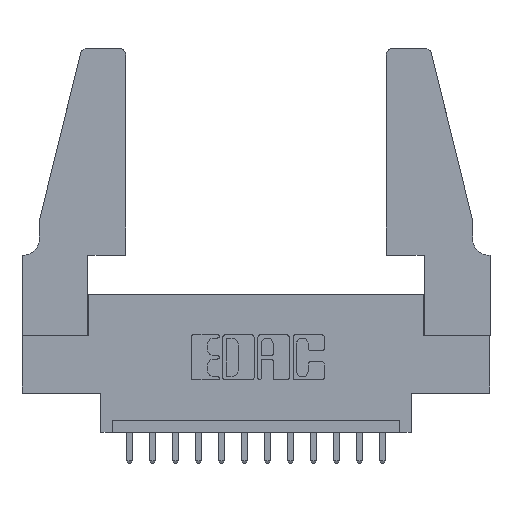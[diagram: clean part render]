
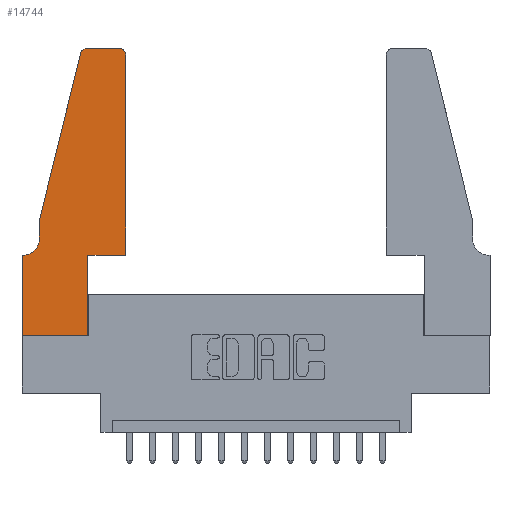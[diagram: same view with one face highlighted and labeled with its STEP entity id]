
A CAD part, top view. The second image highlights one B-rep face of the part: STEP entity #14744.
In plain terms, the highlighted planar face has unit normal (0, 0, 1).
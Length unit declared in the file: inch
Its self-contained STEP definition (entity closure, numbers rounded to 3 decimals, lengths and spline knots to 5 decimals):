
#138 = DIRECTION ( 'NONE',  ( 0., 0., 1. ) ) ;
#202 = ORIENTED_EDGE ( 'NONE', *, *, #7635, .T. ) ;
#237 = LINE ( 'NONE', #12779, #1346 ) ;
#288 = AXIS2_PLACEMENT_3D ( 'NONE', #14298, #138, #10239 ) ;
#647 = VECTOR ( 'NONE', #1321, 39.37008 ) ;
#767 = EDGE_CURVE ( 'NONE', #5536, #14315, #11030, .T. ) ;
#823 = DIRECTION ( 'NONE',  ( 0., 0., -1. ) ) ;
#906 = VECTOR ( 'NONE', #11679, 39.37008 ) ;
#923 = CARTESIAN_POINT ( 'NONE',  ( 0.0055, 0.42, 0.37 ) ) ;
#1123 = PLANE ( 'NONE',  #288 ) ;
#1277 = DIRECTION ( 'NONE',  ( -1., 0., 0. ) ) ;
#1321 = DIRECTION ( 'NONE',  ( 0., 1., 0. ) ) ;
#1346 = VECTOR ( 'NONE', #3264, 39.37008 ) ;
#1425 = CARTESIAN_POINT ( 'NONE',  ( 0.4505, 0.35, 0.37 ) ) ;
#1494 = DIRECTION ( 'NONE',  ( 0., 0., 1. ) ) ;
#1525 = DIRECTION ( 'NONE',  ( 1., 0., 0. ) ) ;
#1696 = CARTESIAN_POINT ( 'NONE',  ( 0.0055, 0.35, 0.37 ) ) ;
#1707 = CARTESIAN_POINT ( 'NONE',  ( 0.0755, 0.5, 0.37 ) ) ;
#1732 = AXIS2_PLACEMENT_3D ( 'NONE', #12116, #1494, #11066 ) ;
#1877 = VERTEX_POINT ( 'NONE', #15377 ) ;
#1930 = DIRECTION ( 'NONE',  ( -1., 0., 0. ) ) ;
#2265 = EDGE_CURVE ( 'NONE', #14378, #5536, #12870, .T. ) ;
#2634 = AXIS2_PLACEMENT_3D ( 'NONE', #923, #823, #1930 ) ;
#2693 = EDGE_CURVE ( 'NONE', #3538, #1877, #11007, .T. ) ;
#2780 = CARTESIAN_POINT ( 'NONE',  ( 0., 0., 0.37 ) ) ;
#2861 = VECTOR ( 'NONE', #1277, 39.37008 ) ;
#2972 = CARTESIAN_POINT ( 'NONE',  ( 0., 0., 0.37 ) ) ;
#3026 = CARTESIAN_POINT ( 'NONE',  ( 0.25487, 1.22718, 0.37 ) ) ;
#3035 = ORIENTED_EDGE ( 'NONE', *, *, #10656, .T. ) ;
#3264 = DIRECTION ( 'NONE',  ( 0., -1., 0. ) ) ;
#3538 = VERTEX_POINT ( 'NONE', #13537 ) ;
#4671 = CARTESIAN_POINT ( 'NONE',  ( 0.2865, 0.35, 0.37 ) ) ;
#4835 = CARTESIAN_POINT ( 'NONE',  ( 0.2865, 0., 0.37 ) ) ;
#4898 = ORIENTED_EDGE ( 'NONE', *, *, #13593, .T. ) ;
#5026 = VERTEX_POINT ( 'NONE', #4835 ) ;
#5220 = CARTESIAN_POINT ( 'NONE',  ( 0.4505, 0.35, 0.37 ) ) ;
#5362 = ORIENTED_EDGE ( 'NONE', *, *, #5808, .T. ) ;
#5449 = DIRECTION ( 'NONE',  ( -0.239, -0.971, 0. ) ) ;
#5536 = VERTEX_POINT ( 'NONE', #5220 ) ;
#5580 = VERTEX_POINT ( 'NONE', #10053 ) ;
#5808 = EDGE_CURVE ( 'NONE', #6667, #7899, #237, .T. ) ;
#5862 = DIRECTION ( 'NONE',  ( 0., 1., 0. ) ) ;
#6001 = LINE ( 'NONE', #6035, #2861 ) ;
#6035 = CARTESIAN_POINT ( 'NONE',  ( 0.2605, 1.25, 0.37 ) ) ;
#6037 = EDGE_CURVE ( 'NONE', #7899, #5026, #14707, .T. ) ;
#6152 = ORIENTED_EDGE ( 'NONE', *, *, #15047, .T. ) ;
#6179 = VECTOR ( 'NONE', #8669, 39.37008 ) ;
#6399 = ORIENTED_EDGE ( 'NONE', *, *, #11668, .T. ) ;
#6403 = DIRECTION ( 'NONE',  ( 0., -1., 0. ) ) ;
#6667 = VERTEX_POINT ( 'NONE', #8924 ) ;
#6786 = VERTEX_POINT ( 'NONE', #1696 ) ;
#6943 = EDGE_CURVE ( 'NONE', #6786, #6667, #14860, .T. ) ;
#7615 = VECTOR ( 'NONE', #13371, 39.37008 ) ;
#7635 = EDGE_CURVE ( 'NONE', #9063, #3538, #10534, .T. ) ;
#7836 = ORIENTED_EDGE ( 'NONE', *, *, #6943, .T. ) ;
#7899 = VERTEX_POINT ( 'NONE', #2972 ) ;
#7925 = VECTOR ( 'NONE', #5862, 39.37008 ) ;
#8066 = CARTESIAN_POINT ( 'NONE',  ( 0.2865, 0.35, 0.37 ) ) ;
#8188 = CIRCLE ( 'NONE', #1732, 0.03 ) ;
#8527 = VECTOR ( 'NONE', #5449, 39.37008 ) ;
#8647 = ORIENTED_EDGE ( 'NONE', *, *, #2265, .T. ) ;
#8669 = DIRECTION ( 'NONE',  ( 1., 0., 0. ) ) ;
#8775 = CARTESIAN_POINT ( 'NONE',  ( 0.4505, 0.35, 0.37 ) ) ;
#8826 = AXIS2_PLACEMENT_3D ( 'NONE', #12973, #9704, #1525 ) ;
#8898 = ORIENTED_EDGE ( 'NONE', *, *, #6037, .T. ) ;
#8924 = CARTESIAN_POINT ( 'NONE',  ( 0., 0.35, 0.37 ) ) ;
#9063 = VERTEX_POINT ( 'NONE', #3026 ) ;
#9704 = DIRECTION ( 'NONE',  ( 0., 0., 1. ) ) ;
#10053 = CARTESIAN_POINT ( 'NONE',  ( 0.4205, 1.25, 0.37 ) ) ;
#10239 = DIRECTION ( 'NONE',  ( 1., 0., 0. ) ) ;
#10513 = EDGE_LOOP ( 'NONE', ( #6152, #4898, #202, #10596, #6399, #7836, #5362, #8898, #10726, #8647, #12332, #3035 ) ) ;
#10534 = LINE ( 'NONE', #15147, #8527 ) ;
#10596 = ORIENTED_EDGE ( 'NONE', *, *, #2693, .T. ) ;
#10633 = VECTOR ( 'NONE', #6403, 39.37008 ) ;
#10656 = EDGE_CURVE ( 'NONE', #14315, #5580, #8188, .T. ) ;
#10726 = ORIENTED_EDGE ( 'NONE', *, *, #12253, .T. ) ;
#11007 = LINE ( 'NONE', #1707, #10633 ) ;
#11030 = LINE ( 'NONE', #1425, #647 ) ;
#11066 = DIRECTION ( 'NONE',  ( 1., 0., 0. ) ) ;
#11668 = EDGE_CURVE ( 'NONE', #1877, #6786, #14659, .T. ) ;
#11679 = DIRECTION ( 'NONE',  ( -1., 0., 0. ) ) ;
#12116 = CARTESIAN_POINT ( 'NONE',  ( 0.4205, 1.22, 0.37 ) ) ;
#12253 = EDGE_CURVE ( 'NONE', #5026, #14378, #12751, .T. ) ;
#12309 = CARTESIAN_POINT ( 'NONE',  ( 0.284, 1.25, 0.37 ) ) ;
#12332 = ORIENTED_EDGE ( 'NONE', *, *, #767, .T. ) ;
#12751 = LINE ( 'NONE', #4671, #7925 ) ;
#12779 = CARTESIAN_POINT ( 'NONE',  ( 0., 0., 0.37 ) ) ;
#12870 = LINE ( 'NONE', #8775, #6179 ) ;
#12973 = CARTESIAN_POINT ( 'NONE',  ( 0.284, 1.22, 0.37 ) ) ;
#12985 = VERTEX_POINT ( 'NONE', #12309 ) ;
#13285 = CIRCLE ( 'NONE', #8826, 0.03 ) ;
#13371 = DIRECTION ( 'NONE',  ( 1., 0., 0. ) ) ;
#13537 = CARTESIAN_POINT ( 'NONE',  ( 0.0755, 0.5, 0.37 ) ) ;
#13593 = EDGE_CURVE ( 'NONE', #12985, #9063, #13285, .T. ) ;
#13914 = CARTESIAN_POINT ( 'NONE',  ( 0.0755, 0.35, 0.37 ) ) ;
#14298 = CARTESIAN_POINT ( 'NONE',  ( 0., 0.35, 0.37 ) ) ;
#14315 = VERTEX_POINT ( 'NONE', #14656 ) ;
#14378 = VERTEX_POINT ( 'NONE', #8066 ) ;
#14656 = CARTESIAN_POINT ( 'NONE',  ( 0.4505, 1.22, 0.37 ) ) ;
#14659 = CIRCLE ( 'NONE', #2634, 0.07 ) ;
#14707 = LINE ( 'NONE', #2780, #7615 ) ;
#14744 = ADVANCED_FACE ( 'NONE', ( #15324 ), #1123, .T. ) ;
#14860 = LINE ( 'NONE', #13914, #906 ) ;
#15047 = EDGE_CURVE ( 'NONE', #5580, #12985, #6001, .T. ) ;
#15147 = CARTESIAN_POINT ( 'NONE',  ( 0.0755, 0.5, 0.37 ) ) ;
#15324 = FACE_OUTER_BOUND ( 'NONE', #10513, .T. ) ;
#15377 = CARTESIAN_POINT ( 'NONE',  ( 0.0755, 0.42, 0.37 ) ) ;
